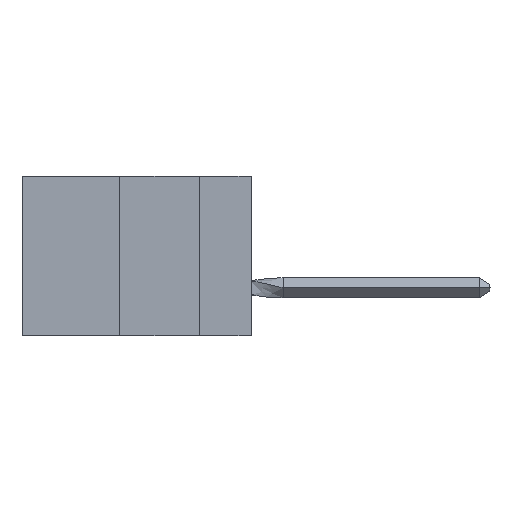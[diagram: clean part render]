
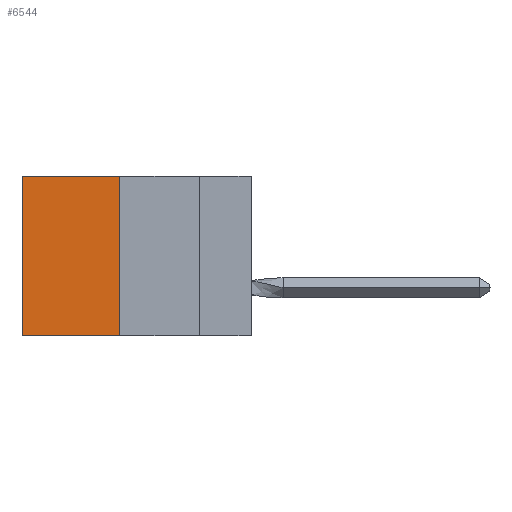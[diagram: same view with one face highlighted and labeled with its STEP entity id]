
A CAD part, left-side view. The second image highlights one B-rep face of the part: STEP entity #6544.
In plain terms, the highlighted planar face has unit normal (-1, 0, 0).
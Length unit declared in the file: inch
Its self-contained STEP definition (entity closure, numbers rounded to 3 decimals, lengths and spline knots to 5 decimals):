
#2134 = EDGE_CURVE ( 'NONE', #10339, #14507, #16915, .T. ) ;
#3077 = VERTEX_POINT ( 'NONE', #5332 ) ;
#3480 = CARTESIAN_POINT ( 'NONE',  ( 0.305, 0.413, -0.5 ) ) ;
#3798 = CARTESIAN_POINT ( 'NONE',  ( 0.305, 0.413, -0.5 ) ) ;
#4268 = VECTOR ( 'NONE', #11753, 39.37008 ) ;
#4649 = EDGE_CURVE ( 'NONE', #14920, #3077, #16521, .T. ) ;
#4751 = CARTESIAN_POINT ( 'NONE',  ( 0.305, 0.413, 0. ) ) ;
#4801 = CARTESIAN_POINT ( 'NONE',  ( 0.305, 0.413, 0. ) ) ;
#5332 = CARTESIAN_POINT ( 'NONE',  ( 0.305, 0.413, -0.5 ) ) ;
#5923 = PLANE ( 'NONE',  #10559 ) ;
#6115 = DIRECTION ( 'NONE',  ( 0., 1., 0. ) ) ;
#6477 = CARTESIAN_POINT ( 'NONE',  ( 0.305, 0.72, -0.5 ) ) ;
#6544 = ADVANCED_FACE ( 'NONE', ( #6719 ), #5923, .F. ) ;
#6719 = FACE_OUTER_BOUND ( 'NONE', #10262, .T. ) ;
#7277 = CARTESIAN_POINT ( 'NONE',  ( 0.305, 0.413, -0.5 ) ) ;
#7676 = ORIENTED_EDGE ( 'NONE', *, *, #9589, .F. ) ;
#9589 = EDGE_CURVE ( 'NONE', #3077, #14507, #12777, .T. ) ;
#10262 = EDGE_LOOP ( 'NONE', ( #17081, #7676, #14293, #15552 ) ) ;
#10339 = VERTEX_POINT ( 'NONE', #17546 ) ;
#10559 = AXIS2_PLACEMENT_3D ( 'NONE', #7277, #14105, #15461 ) ;
#11662 = DIRECTION ( 'NONE',  ( 0., 0., -1. ) ) ;
#11753 = DIRECTION ( 'NONE',  ( 0., 1., 0. ) ) ;
#11849 = VECTOR ( 'NONE', #14672, 39.37008 ) ;
#12063 = EDGE_CURVE ( 'NONE', #14920, #10339, #13760, .T. ) ;
#12777 = LINE ( 'NONE', #3480, #4268 ) ;
#13760 = LINE ( 'NONE', #4801, #15241 ) ;
#14105 = DIRECTION ( 'NONE',  ( 1., 0., 0. ) ) ;
#14293 = ORIENTED_EDGE ( 'NONE', *, *, #4649, .F. ) ;
#14507 = VERTEX_POINT ( 'NONE', #6477 ) ;
#14672 = DIRECTION ( 'NONE',  ( 0., 0., -1. ) ) ;
#14920 = VERTEX_POINT ( 'NONE', #4751 ) ;
#15241 = VECTOR ( 'NONE', #6115, 39.37008 ) ;
#15255 = VECTOR ( 'NONE', #11662, 39.37008 ) ;
#15461 = DIRECTION ( 'NONE',  ( 0., 0., -1. ) ) ;
#15552 = ORIENTED_EDGE ( 'NONE', *, *, #12063, .T. ) ;
#16521 = LINE ( 'NONE', #3798, #11849 ) ;
#16915 = LINE ( 'NONE', #16977, #15255 ) ;
#16977 = CARTESIAN_POINT ( 'NONE',  ( 0.305, 0.72, -0.5 ) ) ;
#17081 = ORIENTED_EDGE ( 'NONE', *, *, #2134, .T. ) ;
#17546 = CARTESIAN_POINT ( 'NONE',  ( 0.305, 0.72, 0. ) ) ;
